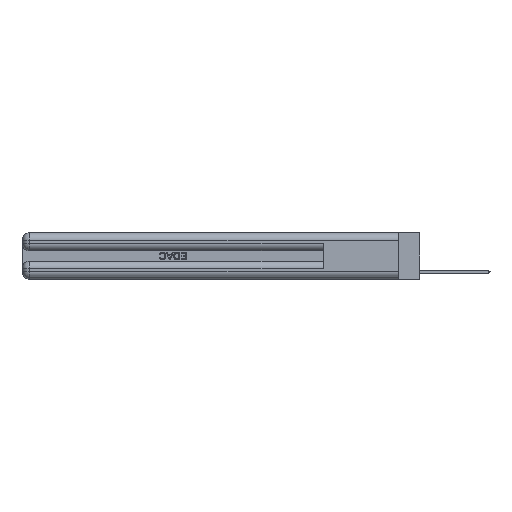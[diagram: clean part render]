
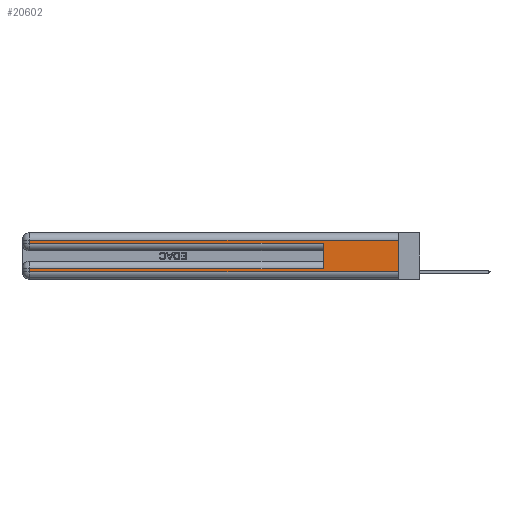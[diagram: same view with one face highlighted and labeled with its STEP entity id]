
A CAD part, left-side view. The second image highlights one B-rep face of the part: STEP entity #20602.
In plain terms, the highlighted planar face has unit normal (-1, 0, 0).
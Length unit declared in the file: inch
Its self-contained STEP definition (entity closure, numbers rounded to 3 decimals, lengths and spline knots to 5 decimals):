
#329 = VERTEX_POINT ( 'NONE', #29623 ) ;
#814 = EDGE_CURVE ( 'NONE', #329, #18252, #6543, .T. ) ;
#1019 = CARTESIAN_POINT ( 'NONE',  ( 0., 0., 0.37 ) ) ;
#1659 = VERTEX_POINT ( 'NONE', #23649 ) ;
#1810 = DIRECTION ( 'NONE',  ( 0., 0., -1. ) ) ;
#1865 = VECTOR ( 'NONE', #28556, 39.37008 ) ;
#2015 = CARTESIAN_POINT ( 'NONE',  ( 0., 2.94, 0.37 ) ) ;
#2093 = VERTEX_POINT ( 'NONE', #4675 ) ;
#3515 = LINE ( 'NONE', #23059, #12874 ) ;
#4091 = CARTESIAN_POINT ( 'NONE',  ( 0., 2.94, 0.37 ) ) ;
#4675 = CARTESIAN_POINT ( 'NONE',  ( 0., 2.94, 0.285 ) ) ;
#5004 = CARTESIAN_POINT ( 'NONE',  ( 0., 0., 0.31 ) ) ;
#5112 = EDGE_CURVE ( 'NONE', #28708, #329, #5536, .T. ) ;
#5536 = LINE ( 'NONE', #2015, #21952 ) ;
#5672 = VECTOR ( 'NONE', #16568, 39.37008 ) ;
#5720 = DIRECTION ( 'NONE',  ( 0., 1., 0. ) ) ;
#6543 = LINE ( 'NONE', #8230, #1865 ) ;
#6920 = VECTOR ( 'NONE', #5720, 39.37008 ) ;
#7130 = ORIENTED_EDGE ( 'NONE', *, *, #13042, .F. ) ;
#7187 = ORIENTED_EDGE ( 'NONE', *, *, #814, .T. ) ;
#7246 = LINE ( 'NONE', #4091, #13076 ) ;
#8230 = CARTESIAN_POINT ( 'NONE',  ( 0., 0., 0.06 ) ) ;
#8264 = AXIS2_PLACEMENT_3D ( 'NONE', #17348, #17679, #27255 ) ;
#10201 = CARTESIAN_POINT ( 'NONE',  ( 0., 2.94, 0.085 ) ) ;
#10535 = DIRECTION ( 'NONE',  ( 0., 1., 0. ) ) ;
#10564 = VERTEX_POINT ( 'NONE', #30636 ) ;
#10681 = VERTEX_POINT ( 'NONE', #5004 ) ;
#12288 = VECTOR ( 'NONE', #21534, 39.37008 ) ;
#12874 = VECTOR ( 'NONE', #10535, 39.37008 ) ;
#13042 = EDGE_CURVE ( 'NONE', #10564, #21259, #15964, .T. ) ;
#13076 = VECTOR ( 'NONE', #22295, 39.37008 ) ;
#14664 = LINE ( 'NONE', #1019, #5672 ) ;
#14755 = PLANE ( 'NONE',  #8264 ) ;
#14963 = EDGE_CURVE ( 'NONE', #10681, #18252, #14664, .T. ) ;
#15964 = LINE ( 'NONE', #21357, #19470 ) ;
#16437 = EDGE_CURVE ( 'NONE', #10564, #28708, #3515, .T. ) ;
#16568 = DIRECTION ( 'NONE',  ( 0., 0., -1. ) ) ;
#17348 = CARTESIAN_POINT ( 'NONE',  ( 0., 0., 0.37 ) ) ;
#17484 = ORIENTED_EDGE ( 'NONE', *, *, #5112, .T. ) ;
#17679 = DIRECTION ( 'NONE',  ( 1., 0., 0. ) ) ;
#18252 = VERTEX_POINT ( 'NONE', #21023 ) ;
#19470 = VECTOR ( 'NONE', #29570, 39.37008 ) ;
#19531 = ORIENTED_EDGE ( 'NONE', *, *, #16437, .T. ) ;
#20388 = EDGE_CURVE ( 'NONE', #2093, #21259, #22432, .T. ) ;
#20602 = ADVANCED_FACE ( 'NONE', ( #29846 ), #14755, .F. ) ;
#20886 = EDGE_LOOP ( 'NONE', ( #24296, #21615, #31844, #26765, #7130, #19531, #17484, #7187 ) ) ;
#21023 = CARTESIAN_POINT ( 'NONE',  ( 0., 0., 0.06 ) ) ;
#21259 = VERTEX_POINT ( 'NONE', #27519 ) ;
#21357 = CARTESIAN_POINT ( 'NONE',  ( 0., 0.6, 0.145 ) ) ;
#21534 = DIRECTION ( 'NONE',  ( 0., -1., 0. ) ) ;
#21615 = ORIENTED_EDGE ( 'NONE', *, *, #24822, .T. ) ;
#21952 = VECTOR ( 'NONE', #1810, 39.37008 ) ;
#22295 = DIRECTION ( 'NONE',  ( 0., 0., -1. ) ) ;
#22432 = LINE ( 'NONE', #23871, #12288 ) ;
#23059 = CARTESIAN_POINT ( 'NONE',  ( 0., 0., 0.085 ) ) ;
#23412 = CARTESIAN_POINT ( 'NONE',  ( 0., 0., 0.31 ) ) ;
#23649 = CARTESIAN_POINT ( 'NONE',  ( 0., 2.94, 0.31 ) ) ;
#23871 = CARTESIAN_POINT ( 'NONE',  ( 0., 0., 0.285 ) ) ;
#24296 = ORIENTED_EDGE ( 'NONE', *, *, #14963, .F. ) ;
#24822 = EDGE_CURVE ( 'NONE', #10681, #1659, #29988, .T. ) ;
#25826 = EDGE_CURVE ( 'NONE', #1659, #2093, #7246, .T. ) ;
#26765 = ORIENTED_EDGE ( 'NONE', *, *, #20388, .T. ) ;
#27255 = DIRECTION ( 'NONE',  ( 0., 0., -1. ) ) ;
#27519 = CARTESIAN_POINT ( 'NONE',  ( 0., 0.6, 0.285 ) ) ;
#28556 = DIRECTION ( 'NONE',  ( 0., -1., 0. ) ) ;
#28708 = VERTEX_POINT ( 'NONE', #10201 ) ;
#29570 = DIRECTION ( 'NONE',  ( 0., 0., 1. ) ) ;
#29623 = CARTESIAN_POINT ( 'NONE',  ( 0., 2.94, 0.06 ) ) ;
#29846 = FACE_OUTER_BOUND ( 'NONE', #20886, .T. ) ;
#29988 = LINE ( 'NONE', #23412, #6920 ) ;
#30636 = CARTESIAN_POINT ( 'NONE',  ( 0., 0.6, 0.085 ) ) ;
#31844 = ORIENTED_EDGE ( 'NONE', *, *, #25826, .T. ) ;
